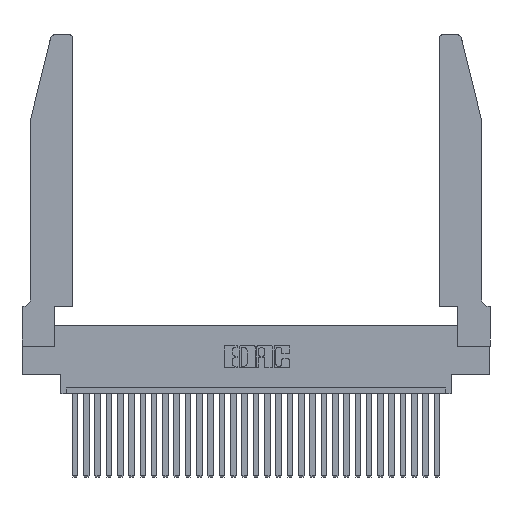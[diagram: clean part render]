
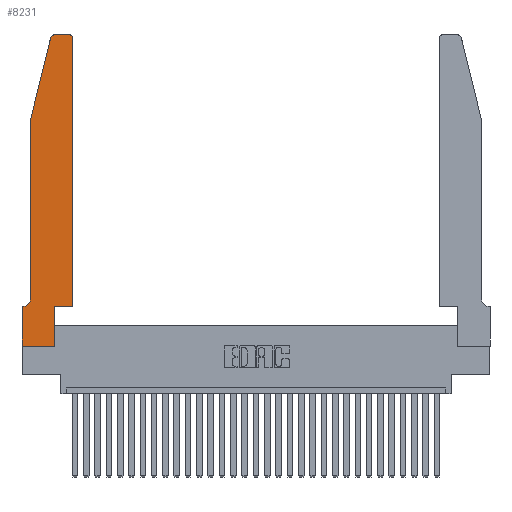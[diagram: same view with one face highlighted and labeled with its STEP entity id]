
A CAD part, top view. The second image highlights one B-rep face of the part: STEP entity #8231.
In plain terms, the highlighted planar face has unit normal (0, 0, 1).
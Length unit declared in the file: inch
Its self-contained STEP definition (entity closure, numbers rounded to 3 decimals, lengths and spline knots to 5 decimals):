
#1043 = EDGE_CURVE ( 'NONE', #15762, #27929, #25327, .T. ) ;
#1344 = DIRECTION ( 'NONE',  ( 0., 0., 1. ) ) ;
#1507 = FACE_OUTER_BOUND ( 'NONE', #20002, .T. ) ;
#2512 = EDGE_CURVE ( 'NONE', #27929, #12247, #16699, .T. ) ;
#3113 = VERTEX_POINT ( 'NONE', #20730 ) ;
#3667 = DIRECTION ( 'NONE',  ( 1., 0., 0. ) ) ;
#3746 = DIRECTION ( 'NONE',  ( 1., 0., 0. ) ) ;
#4500 = DIRECTION ( 'NONE',  ( 0., -1., 0. ) ) ;
#4863 = DIRECTION ( 'NONE',  ( -1., 0., 0. ) ) ;
#5448 = VERTEX_POINT ( 'NONE', #18708 ) ;
#5752 = VECTOR ( 'NONE', #13998, 39.37008 ) ;
#6632 = VERTEX_POINT ( 'NONE', #12265 ) ;
#7057 = VERTEX_POINT ( 'NONE', #17032 ) ;
#7245 = VERTEX_POINT ( 'NONE', #9582 ) ;
#7349 = CARTESIAN_POINT ( 'NONE',  ( 0.284, 2.72, 0.37 ) ) ;
#7426 = ORIENTED_EDGE ( 'NONE', *, *, #2512, .T. ) ;
#8201 = VECTOR ( 'NONE', #4500, 39.37008 ) ;
#8231 = ADVANCED_FACE ( 'NONE', ( #1507 ), #12857, .T. ) ;
#8963 = LINE ( 'NONE', #18426, #10046 ) ;
#9098 = CARTESIAN_POINT ( 'NONE',  ( 0.284, 2.75, 0.37 ) ) ;
#9149 = CARTESIAN_POINT ( 'NONE',  ( 0.0755, 2., 0.37 ) ) ;
#9319 = CARTESIAN_POINT ( 'NONE',  ( 0.4505, 0.35, 0.37 ) ) ;
#9406 = ORIENTED_EDGE ( 'NONE', *, *, #1043, .T. ) ;
#9582 = CARTESIAN_POINT ( 'NONE',  ( 0.25487, 2.72718, 0.37 ) ) ;
#9746 = DIRECTION ( 'NONE',  ( 1., 0., 0. ) ) ;
#9983 = DIRECTION ( 'NONE',  ( -1., 0., 0. ) ) ;
#10046 = VECTOR ( 'NONE', #22752, 39.37008 ) ;
#10281 = LINE ( 'NONE', #30212, #21122 ) ;
#10306 = VECTOR ( 'NONE', #23535, 39.37008 ) ;
#10781 = VERTEX_POINT ( 'NONE', #23860 ) ;
#11496 = EDGE_CURVE ( 'NONE', #3113, #12489, #13602, .T. ) ;
#11520 = ORIENTED_EDGE ( 'NONE', *, *, #11496, .T. ) ;
#11749 = VECTOR ( 'NONE', #16542, 39.37008 ) ;
#11872 = CARTESIAN_POINT ( 'NONE',  ( 0.2865, 0., 0.37 ) ) ;
#12081 = LINE ( 'NONE', #9319, #5752 ) ;
#12247 = VERTEX_POINT ( 'NONE', #21248 ) ;
#12265 = CARTESIAN_POINT ( 'NONE',  ( 0., 0., 0.37 ) ) ;
#12489 = VERTEX_POINT ( 'NONE', #22799 ) ;
#12556 = DIRECTION ( 'NONE',  ( 1., 0., 0. ) ) ;
#12659 = CARTESIAN_POINT ( 'NONE',  ( 0.4205, 2.72, 0.37 ) ) ;
#12731 = VECTOR ( 'NONE', #29341, 39.37008 ) ;
#12857 = PLANE ( 'NONE',  #30135 ) ;
#13071 = CARTESIAN_POINT ( 'NONE',  ( 0., 0.35, 0.37 ) ) ;
#13345 = EDGE_CURVE ( 'NONE', #12489, #10781, #12081, .T. ) ;
#13385 = CARTESIAN_POINT ( 'NONE',  ( 0., 0., 0.37 ) ) ;
#13602 = LINE ( 'NONE', #19320, #18476 ) ;
#13682 = ORIENTED_EDGE ( 'NONE', *, *, #30003, .T. ) ;
#13998 = DIRECTION ( 'NONE',  ( 0., 1., 0. ) ) ;
#14435 = EDGE_CURVE ( 'NONE', #7057, #6632, #20572, .T. ) ;
#14638 = DIRECTION ( 'NONE',  ( 1., 0., 0. ) ) ;
#15762 = VERTEX_POINT ( 'NONE', #19872 ) ;
#16362 = CIRCLE ( 'NONE', #28507, 0.03 ) ;
#16542 = DIRECTION ( 'NONE',  ( 0., 1., 0. ) ) ;
#16699 = CIRCLE ( 'NONE', #29645, 0.07 ) ;
#16988 = CARTESIAN_POINT ( 'NONE',  ( 0.0055, 0.42, 0.37 ) ) ;
#17032 = CARTESIAN_POINT ( 'NONE',  ( 0., 0.35, 0.37 ) ) ;
#17375 = EDGE_CURVE ( 'NONE', #12247, #7057, #10281, .T. ) ;
#18144 = ORIENTED_EDGE ( 'NONE', *, *, #26882, .T. ) ;
#18426 = CARTESIAN_POINT ( 'NONE',  ( 0.0755, 2., 0.37 ) ) ;
#18476 = VECTOR ( 'NONE', #14638, 39.37008 ) ;
#18708 = CARTESIAN_POINT ( 'NONE',  ( 0.4205, 2.75, 0.37 ) ) ;
#19114 = CARTESIAN_POINT ( 'NONE',  ( 0.2865, 0.35, 0.37 ) ) ;
#19320 = CARTESIAN_POINT ( 'NONE',  ( 0.4505, 0.35, 0.37 ) ) ;
#19872 = CARTESIAN_POINT ( 'NONE',  ( 0.0755, 2., 0.37 ) ) ;
#20002 = EDGE_LOOP ( 'NONE', ( #26101, #22952, #18144, #9406, #7426, #20200, #28181, #24587, #13682, #11520, #27441, #30362 ) ) ;
#20200 = ORIENTED_EDGE ( 'NONE', *, *, #17375, .T. ) ;
#20516 = EDGE_CURVE ( 'NONE', #6632, #30155, #22678, .T. ) ;
#20572 = LINE ( 'NONE', #23628, #12731 ) ;
#20730 = CARTESIAN_POINT ( 'NONE',  ( 0.2865, 0.35, 0.37 ) ) ;
#21122 = VECTOR ( 'NONE', #4863, 39.37008 ) ;
#21212 = VECTOR ( 'NONE', #3667, 39.37008 ) ;
#21248 = CARTESIAN_POINT ( 'NONE',  ( 0.0055, 0.35, 0.37 ) ) ;
#21614 = DIRECTION ( 'NONE',  ( 0., 0., 1. ) ) ;
#22225 = CARTESIAN_POINT ( 'NONE',  ( 0.0755, 0.42, 0.37 ) ) ;
#22678 = LINE ( 'NONE', #13385, #21212 ) ;
#22752 = DIRECTION ( 'NONE',  ( -0.239, -0.971, 0. ) ) ;
#22799 = CARTESIAN_POINT ( 'NONE',  ( 0.4505, 0.35, 0.37 ) ) ;
#22915 = LINE ( 'NONE', #19114, #11749 ) ;
#22952 = ORIENTED_EDGE ( 'NONE', *, *, #24142, .T. ) ;
#23535 = DIRECTION ( 'NONE',  ( -1., 0., 0. ) ) ;
#23628 = CARTESIAN_POINT ( 'NONE',  ( 0., 0., 0.37 ) ) ;
#23860 = CARTESIAN_POINT ( 'NONE',  ( 0.4505, 2.72, 0.37 ) ) ;
#24142 = EDGE_CURVE ( 'NONE', #25885, #7245, #30679, .T. ) ;
#24223 = DIRECTION ( 'NONE',  ( 0., 0., -1. ) ) ;
#24587 = ORIENTED_EDGE ( 'NONE', *, *, #20516, .T. ) ;
#25327 = LINE ( 'NONE', #9149, #8201 ) ;
#25885 = VERTEX_POINT ( 'NONE', #9098 ) ;
#26101 = ORIENTED_EDGE ( 'NONE', *, *, #28760, .T. ) ;
#26693 = LINE ( 'NONE', #30605, #10306 ) ;
#26882 = EDGE_CURVE ( 'NONE', #7245, #15762, #8963, .T. ) ;
#27441 = ORIENTED_EDGE ( 'NONE', *, *, #13345, .T. ) ;
#27782 = EDGE_CURVE ( 'NONE', #10781, #5448, #16362, .T. ) ;
#27929 = VERTEX_POINT ( 'NONE', #22225 ) ;
#28181 = ORIENTED_EDGE ( 'NONE', *, *, #14435, .T. ) ;
#28507 = AXIS2_PLACEMENT_3D ( 'NONE', #12659, #29101, #12556 ) ;
#28760 = EDGE_CURVE ( 'NONE', #5448, #25885, #26693, .T. ) ;
#29101 = DIRECTION ( 'NONE',  ( 0., 0., 1. ) ) ;
#29341 = DIRECTION ( 'NONE',  ( 0., -1., 0. ) ) ;
#29633 = AXIS2_PLACEMENT_3D ( 'NONE', #7349, #21614, #9746 ) ;
#29645 = AXIS2_PLACEMENT_3D ( 'NONE', #16988, #24223, #9983 ) ;
#30003 = EDGE_CURVE ( 'NONE', #30155, #3113, #22915, .T. ) ;
#30135 = AXIS2_PLACEMENT_3D ( 'NONE', #13071, #1344, #3746 ) ;
#30155 = VERTEX_POINT ( 'NONE', #11872 ) ;
#30212 = CARTESIAN_POINT ( 'NONE',  ( 0.0755, 0.35, 0.37 ) ) ;
#30362 = ORIENTED_EDGE ( 'NONE', *, *, #27782, .T. ) ;
#30605 = CARTESIAN_POINT ( 'NONE',  ( 0.2605, 2.75, 0.37 ) ) ;
#30679 = CIRCLE ( 'NONE', #29633, 0.03 ) ;
